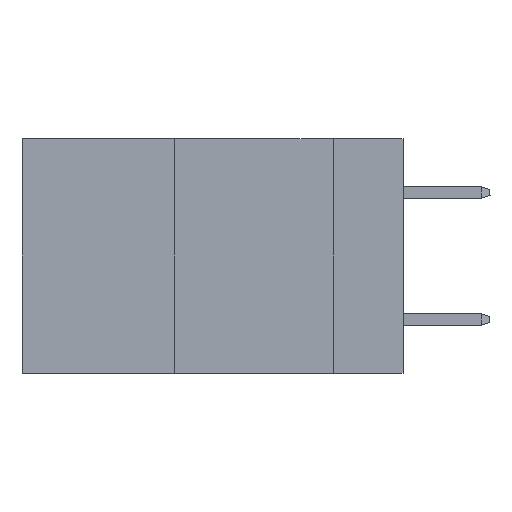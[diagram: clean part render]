
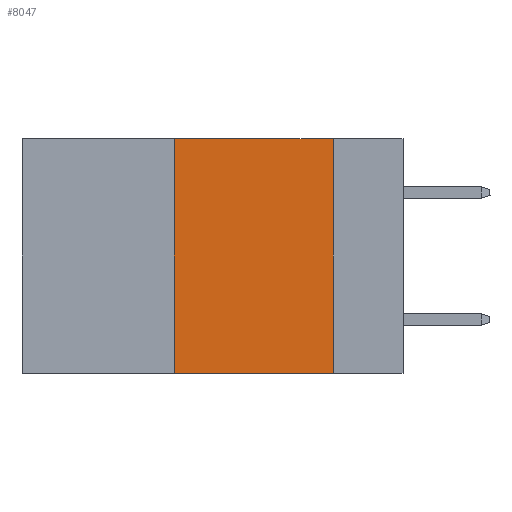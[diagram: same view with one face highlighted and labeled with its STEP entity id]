
A CAD part, left-side view. The second image highlights one B-rep face of the part: STEP entity #8047.
In plain terms, the highlighted planar face has unit normal (-1, 0, 0).
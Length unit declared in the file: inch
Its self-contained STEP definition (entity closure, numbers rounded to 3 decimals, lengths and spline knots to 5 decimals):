
#256 = CARTESIAN_POINT ( 'NONE',  ( 0., 0.11, 0. ) ) ;
#639 = VECTOR ( 'NONE', #9745, 39.37008 ) ;
#2191 = DIRECTION ( 'NONE',  ( 1., 0., 0. ) ) ;
#2348 = ORIENTED_EDGE ( 'NONE', *, *, #30639, .F. ) ;
#3018 = EDGE_LOOP ( 'NONE', ( #20186, #2348, #6320, #23534 ) ) ;
#3605 = CARTESIAN_POINT ( 'NONE',  ( 0., 0.11, -0.37 ) ) ;
#5142 = VECTOR ( 'NONE', #18365, 39.37008 ) ;
#5170 = FACE_OUTER_BOUND ( 'NONE', #3018, .T. ) ;
#6320 = ORIENTED_EDGE ( 'NONE', *, *, #10714, .F. ) ;
#8047 = ADVANCED_FACE ( 'NONE', ( #5170 ), #17225, .F. ) ;
#9745 = DIRECTION ( 'NONE',  ( 0., -1., 0. ) ) ;
#9944 = CARTESIAN_POINT ( 'NONE',  ( 0., 0.6, 0. ) ) ;
#9991 = EDGE_CURVE ( 'NONE', #17988, #30593, #33681, .T. ) ;
#10714 = EDGE_CURVE ( 'NONE', #14433, #32514, #15577, .T. ) ;
#14235 = DIRECTION ( 'NONE',  ( 0., 0., -1. ) ) ;
#14433 = VERTEX_POINT ( 'NONE', #19617 ) ;
#14538 = VECTOR ( 'NONE', #27930, 39.37008 ) ;
#15060 = LINE ( 'NONE', #9944, #639 ) ;
#15577 = LINE ( 'NONE', #27439, #5142 ) ;
#17225 = PLANE ( 'NONE',  #26436 ) ;
#17988 = VERTEX_POINT ( 'NONE', #33888 ) ;
#18365 = DIRECTION ( 'NONE',  ( 0., 0., 1. ) ) ;
#19617 = CARTESIAN_POINT ( 'NONE',  ( 0., 0.36, -0.37 ) ) ;
#20186 = ORIENTED_EDGE ( 'NONE', *, *, #9991, .F. ) ;
#21612 = VECTOR ( 'NONE', #23791, 39.37008 ) ;
#23534 = ORIENTED_EDGE ( 'NONE', *, *, #32423, .T. ) ;
#23791 = DIRECTION ( 'NONE',  ( 0., -1., 0. ) ) ;
#25710 = CARTESIAN_POINT ( 'NONE',  ( 0., 0.36, 0. ) ) ;
#26436 = AXIS2_PLACEMENT_3D ( 'NONE', #29301, #2191, #14235 ) ;
#27439 = CARTESIAN_POINT ( 'NONE',  ( 0., 0.36, 0. ) ) ;
#27930 = DIRECTION ( 'NONE',  ( 0., 0., -1. ) ) ;
#29301 = CARTESIAN_POINT ( 'NONE',  ( 0., 0.6, 0. ) ) ;
#30593 = VERTEX_POINT ( 'NONE', #3605 ) ;
#30639 = EDGE_CURVE ( 'NONE', #32514, #17988, #15060, .T. ) ;
#32423 = EDGE_CURVE ( 'NONE', #14433, #30593, #38986, .T. ) ;
#32514 = VERTEX_POINT ( 'NONE', #25710 ) ;
#33681 = LINE ( 'NONE', #256, #14538 ) ;
#33888 = CARTESIAN_POINT ( 'NONE',  ( 0., 0.11, 0. ) ) ;
#38585 = CARTESIAN_POINT ( 'NONE',  ( 0., 0.6, -0.37 ) ) ;
#38986 = LINE ( 'NONE', #38585, #21612 ) ;
